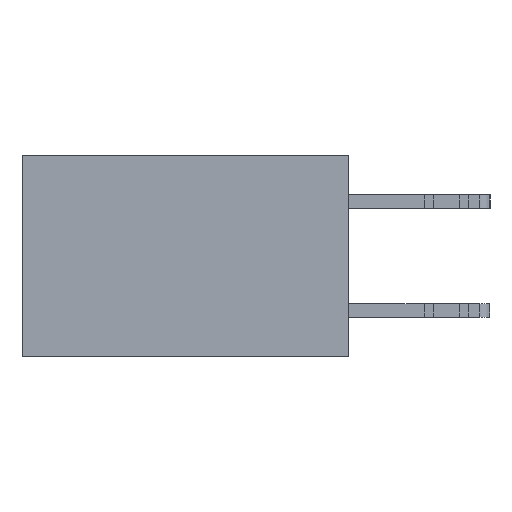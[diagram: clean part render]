
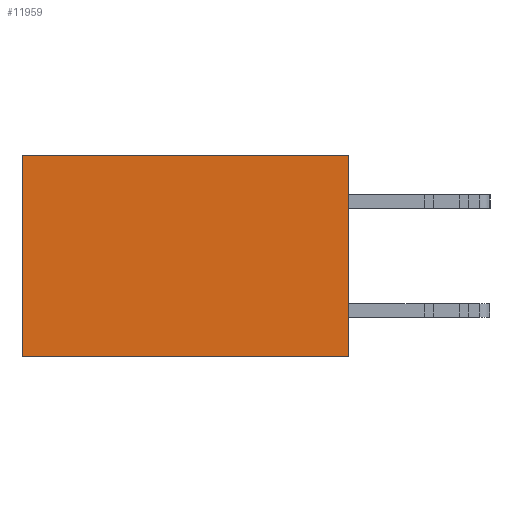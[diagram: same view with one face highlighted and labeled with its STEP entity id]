
A CAD part, left-side view. The second image highlights one B-rep face of the part: STEP entity #11959.
In plain terms, the highlighted planar face has unit normal (-1, 0, 0).
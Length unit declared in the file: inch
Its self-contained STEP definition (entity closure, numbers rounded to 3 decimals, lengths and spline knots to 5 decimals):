
#324 = CARTESIAN_POINT ( 'NONE',  ( 0.2615, 0.6, -0.37 ) ) ;
#409 = EDGE_LOOP ( 'NONE', ( #22921, #8387, #6107, #21942 ) ) ;
#2316 = CARTESIAN_POINT ( 'NONE',  ( 0.2615, 0., -0.37 ) ) ;
#2817 = CARTESIAN_POINT ( 'NONE',  ( 0.2615, 0.6, 0. ) ) ;
#3737 = VECTOR ( 'NONE', #4739, 39.37008 ) ;
#4739 = DIRECTION ( 'NONE',  ( 0., 0., -1. ) ) ;
#5292 = CARTESIAN_POINT ( 'NONE',  ( 0.2615, 0., 0. ) ) ;
#6107 = ORIENTED_EDGE ( 'NONE', *, *, #6196, .F. ) ;
#6196 = EDGE_CURVE ( 'NONE', #13894, #13014, #8448, .T. ) ;
#7082 = DIRECTION ( 'NONE',  ( 0., 0., -1. ) ) ;
#7337 = DIRECTION ( 'NONE',  ( 0., 1., 0. ) ) ;
#7989 = DIRECTION ( 'NONE',  ( 0., 0., -1. ) ) ;
#8116 = VERTEX_POINT ( 'NONE', #2817 ) ;
#8387 = ORIENTED_EDGE ( 'NONE', *, *, #23067, .F. ) ;
#8448 = LINE ( 'NONE', #10870, #3737 ) ;
#9261 = VECTOR ( 'NONE', #15948, 39.37008 ) ;
#9523 = FACE_OUTER_BOUND ( 'NONE', #409, .T. ) ;
#10105 = CARTESIAN_POINT ( 'NONE',  ( 0.2615, 0., -0.37 ) ) ;
#10870 = CARTESIAN_POINT ( 'NONE',  ( 0.2615, 0., -0.37 ) ) ;
#10881 = AXIS2_PLACEMENT_3D ( 'NONE', #17437, #15630, #7989 ) ;
#11036 = CARTESIAN_POINT ( 'NONE',  ( 0.2615, 0.6, -0.37 ) ) ;
#11523 = LINE ( 'NONE', #5292, #24233 ) ;
#11959 = ADVANCED_FACE ( 'NONE', ( #9523 ), #17669, .F. ) ;
#13014 = VERTEX_POINT ( 'NONE', #10105 ) ;
#13894 = VERTEX_POINT ( 'NONE', #18516 ) ;
#15630 = DIRECTION ( 'NONE',  ( 1., 0., 0. ) ) ;
#15948 = DIRECTION ( 'NONE',  ( 0., 1., 0. ) ) ;
#17437 = CARTESIAN_POINT ( 'NONE',  ( 0.2615, 0., -0.37 ) ) ;
#17669 = PLANE ( 'NONE',  #10881 ) ;
#18419 = EDGE_CURVE ( 'NONE', #13894, #8116, #11523, .T. ) ;
#18516 = CARTESIAN_POINT ( 'NONE',  ( 0.2615, 0., 0. ) ) ;
#19623 = EDGE_CURVE ( 'NONE', #8116, #21234, #22620, .T. ) ;
#19752 = LINE ( 'NONE', #2316, #9261 ) ;
#19778 = VECTOR ( 'NONE', #7082, 39.37008 ) ;
#21234 = VERTEX_POINT ( 'NONE', #324 ) ;
#21942 = ORIENTED_EDGE ( 'NONE', *, *, #18419, .T. ) ;
#22620 = LINE ( 'NONE', #11036, #19778 ) ;
#22921 = ORIENTED_EDGE ( 'NONE', *, *, #19623, .T. ) ;
#23067 = EDGE_CURVE ( 'NONE', #13014, #21234, #19752, .T. ) ;
#24233 = VECTOR ( 'NONE', #7337, 39.37008 ) ;
